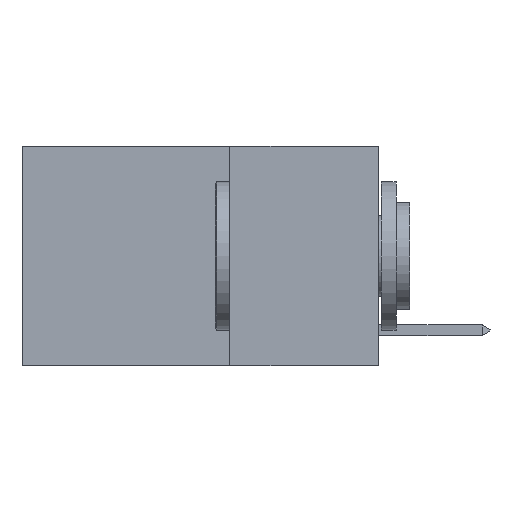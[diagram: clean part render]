
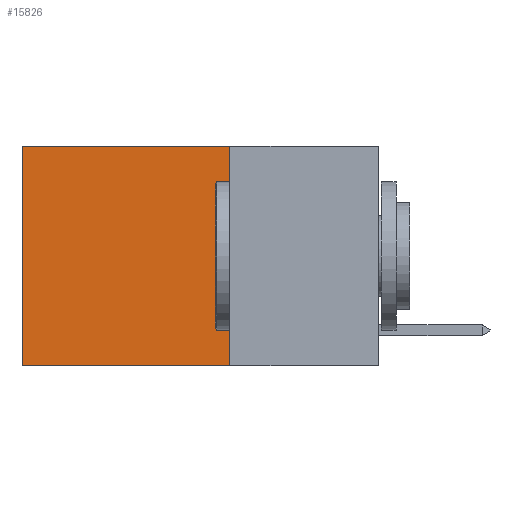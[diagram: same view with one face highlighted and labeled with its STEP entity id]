
A CAD part, left-side view. The second image highlights one B-rep face of the part: STEP entity #15826.
In plain terms, the highlighted planar face has unit normal (-1, 0, 0).
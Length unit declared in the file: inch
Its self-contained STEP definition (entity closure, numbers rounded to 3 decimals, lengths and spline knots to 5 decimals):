
#412 = CARTESIAN_POINT ( 'NONE',  ( 0.2625, 0.25, 0. ) ) ;
#454 = LINE ( 'NONE', #2641, #19478 ) ;
#2322 = DIRECTION ( 'NONE',  ( 0., 1., 0. ) ) ;
#2641 = CARTESIAN_POINT ( 'NONE',  ( 0.2625, 0.25, -0.37 ) ) ;
#3197 = DIRECTION ( 'NONE',  ( 1., 0., 0. ) ) ;
#3262 = EDGE_CURVE ( 'NONE', #20057, #23564, #17516, .T. ) ;
#5832 = AXIS2_PLACEMENT_3D ( 'NONE', #412, #3197, #17046 ) ;
#6660 = DIRECTION ( 'NONE',  ( 0., 0., -1. ) ) ;
#6970 = CARTESIAN_POINT ( 'NONE',  ( 0.2625, 0.25, 0. ) ) ;
#9003 = CARTESIAN_POINT ( 'NONE',  ( 0.2625, 0.25, -0.37 ) ) ;
#9434 = CARTESIAN_POINT ( 'NONE',  ( 0.2625, 0.6, 0. ) ) ;
#10117 = ORIENTED_EDGE ( 'NONE', *, *, #20944, .F. ) ;
#10428 = EDGE_LOOP ( 'NONE', ( #27182, #28010, #10117, #21074 ) ) ;
#10761 = VERTEX_POINT ( 'NONE', #9003 ) ;
#14583 = CARTESIAN_POINT ( 'NONE',  ( 0.2625, 0.25, 0. ) ) ;
#14734 = CARTESIAN_POINT ( 'NONE',  ( 0.2625, 0.25, 0. ) ) ;
#14791 = EDGE_CURVE ( 'NONE', #23564, #21068, #30636, .T. ) ;
#15826 = ADVANCED_FACE ( 'NONE', ( #21706 ), #29103, .F. ) ;
#15865 = VECTOR ( 'NONE', #19690, 39.37008 ) ;
#17046 = DIRECTION ( 'NONE',  ( 0., 0., -1. ) ) ;
#17487 = VECTOR ( 'NONE', #6660, 39.37008 ) ;
#17516 = LINE ( 'NONE', #14734, #15865 ) ;
#18888 = DIRECTION ( 'NONE',  ( 0., 0., -1. ) ) ;
#19478 = VECTOR ( 'NONE', #2322, 39.37008 ) ;
#19614 = EDGE_CURVE ( 'NONE', #10761, #21068, #454, .T. ) ;
#19690 = DIRECTION ( 'NONE',  ( 0., 1., 0. ) ) ;
#20057 = VERTEX_POINT ( 'NONE', #14583 ) ;
#20944 = EDGE_CURVE ( 'NONE', #20057, #10761, #27894, .T. ) ;
#21068 = VERTEX_POINT ( 'NONE', #26194 ) ;
#21074 = ORIENTED_EDGE ( 'NONE', *, *, #3262, .T. ) ;
#21706 = FACE_OUTER_BOUND ( 'NONE', #10428, .T. ) ;
#23564 = VERTEX_POINT ( 'NONE', #30247 ) ;
#26194 = CARTESIAN_POINT ( 'NONE',  ( 0.2625, 0.6, -0.37 ) ) ;
#27182 = ORIENTED_EDGE ( 'NONE', *, *, #14791, .T. ) ;
#27894 = LINE ( 'NONE', #6970, #17487 ) ;
#28010 = ORIENTED_EDGE ( 'NONE', *, *, #19614, .F. ) ;
#28924 = VECTOR ( 'NONE', #18888, 39.37008 ) ;
#29103 = PLANE ( 'NONE',  #5832 ) ;
#30247 = CARTESIAN_POINT ( 'NONE',  ( 0.2625, 0.6, 0. ) ) ;
#30636 = LINE ( 'NONE', #9434, #28924 ) ;
